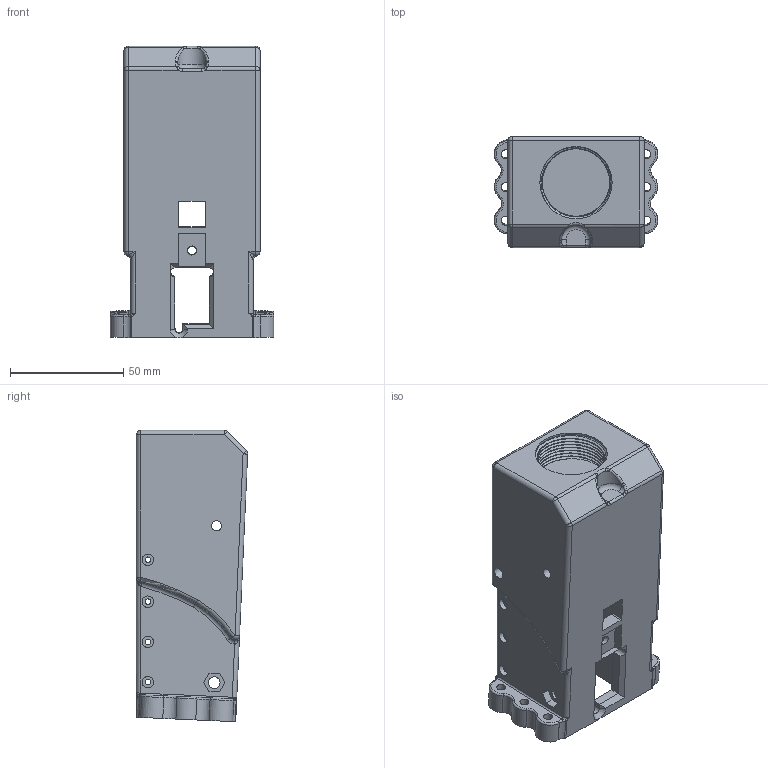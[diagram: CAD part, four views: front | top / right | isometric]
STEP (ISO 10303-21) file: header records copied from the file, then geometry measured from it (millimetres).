
FILE_DESCRIPTION(/* description */ (''),/* implementation_level */ '2;1');
FILE_NAME(/* name */ 'Plastikov v3.1 Rear Receiver AR15 Stock.stp',/* time_stamp */ '2022-03-21T11:51:01-05:00',/* author */ ('johne'),/* organization */ (''),/* preprocessor_version */ 'ST-DEVELOPER v18.1',/* originating_system */ 'Autodesk Inventor 2020',/* authorisation */ '');
FILE_SCHEMA (('AUTOMOTIVE_DESIGN { 1 0 10303 214 3 1 1 }'));
Products named in the file (1): Plastikov v3.1 Rear Receiver AR15 Stock
Bounding box: 72.2 x 49.14 x 128.76 mm (x, y, z)
Volume: 198861 mm3; surface area: 46035.2 mm2
Topology: 1 solids, 17 shells, 321 faces, 741 edges, 456 vertices
Faces by surface type: cylinder 103, plane 95, bspline 72, torus 32, sphere 16, cone 3
Full cylindrical faces by diameter (mm): 2.5 x8, 4 x7, 4.5 x2, 5.08 x8, 5.1 x2, 12 x1, 29.808 x6, 31.903 x1
Entity records: 43205 total; most frequent: CARTESIAN_POINT 35844, ORIENTED_EDGE 1466, DIRECTION 1424, EDGE_CURVE 733, AXIS2_PLACEMENT_3D 573, VERTEX_POINT 456, EDGE_LOOP 373, FACE_OUTER_BOUND 321
